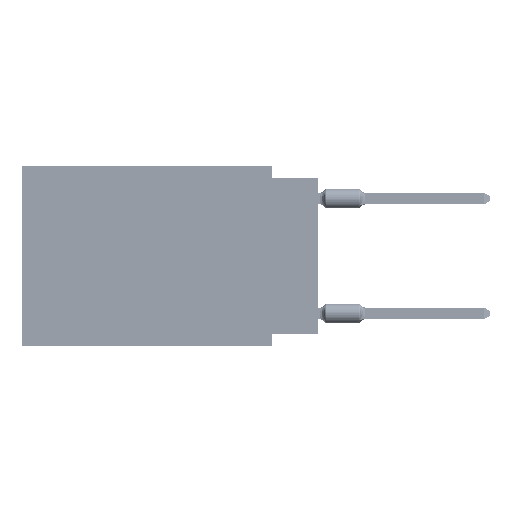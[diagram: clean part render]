
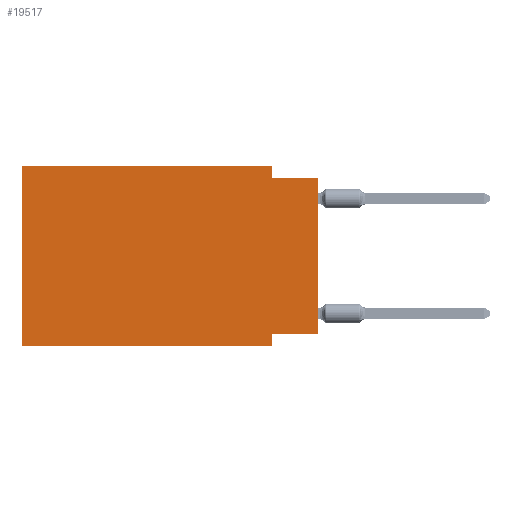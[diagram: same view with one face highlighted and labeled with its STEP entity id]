
A CAD part, left-side view. The second image highlights one B-rep face of the part: STEP entity #19517.
In plain terms, the highlighted planar face has unit normal (-1, 0, 0).
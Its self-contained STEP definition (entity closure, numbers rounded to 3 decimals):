
#997 = CARTESIAN_POINT ( 'NONE',  ( 0., 0., 0. ) ) ;
#1461 = ORIENTED_EDGE ( 'NONE', *, *, #12171, .T. ) ;
#1548 = CARTESIAN_POINT ( 'NONE',  ( 0., 16.383, 0. ) ) ;
#1754 = LINE ( 'NONE', #11423, #20943 ) ;
#3385 = VERTEX_POINT ( 'NONE', #8184 ) ;
#3868 = DIRECTION ( 'NONE',  ( 1., 0., 0. ) ) ;
#5602 = EDGE_CURVE ( 'NONE', #11889, #20168, #49366, .T. ) ;
#5923 = DIRECTION ( 'NONE',  ( 0., 1., 0. ) ) ;
#6121 = EDGE_CURVE ( 'NONE', #3385, #27417, #27793, .T. ) ;
#7916 = ORIENTED_EDGE ( 'NONE', *, *, #41001, .F. ) ;
#8184 = CARTESIAN_POINT ( 'NONE',  ( 0., 0., -9.271 ) ) ;
#9067 = CARTESIAN_POINT ( 'NONE',  ( 0., 16.383, 0. ) ) ;
#9395 = VECTOR ( 'NONE', #56361, 1000. ) ;
#11322 = VERTEX_POINT ( 'NONE', #67606 ) ;
#11423 = CARTESIAN_POINT ( 'NONE',  ( 0., 2.54, 0. ) ) ;
#11850 = CARTESIAN_POINT ( 'NONE',  ( 0., 0., -9.271 ) ) ;
#11889 = VERTEX_POINT ( 'NONE', #1548 ) ;
#12171 = EDGE_CURVE ( 'NONE', #3385, #71257, #22879, .T. ) ;
#13112 = VERTEX_POINT ( 'NONE', #24906 ) ;
#13745 = AXIS2_PLACEMENT_3D ( 'NONE', #41793, #3868, #64391 ) ;
#14829 = EDGE_CURVE ( 'NONE', #13112, #11889, #71295, .T. ) ;
#15281 = ORIENTED_EDGE ( 'NONE', *, *, #58398, .F. ) ;
#17285 = LINE ( 'NONE', #69511, #36307 ) ;
#18370 = DIRECTION ( 'NONE',  ( 0., 0., -1. ) ) ;
#19517 = ADVANCED_FACE ( 'NONE', ( #47333 ), #71661, .F. ) ;
#20168 = VERTEX_POINT ( 'NONE', #47807 ) ;
#20874 = CARTESIAN_POINT ( 'NONE',  ( 0., 16.383, 0. ) ) ;
#20943 = VECTOR ( 'NONE', #40680, 1000. ) ;
#22879 = LINE ( 'NONE', #997, #32936 ) ;
#23630 = CARTESIAN_POINT ( 'NONE',  ( 0., 0., -0.635 ) ) ;
#24906 = CARTESIAN_POINT ( 'NONE',  ( 0., 16.383, -9.906 ) ) ;
#26355 = VECTOR ( 'NONE', #65716, 1000. ) ;
#26816 = ORIENTED_EDGE ( 'NONE', *, *, #5602, .F. ) ;
#27417 = VERTEX_POINT ( 'NONE', #38513 ) ;
#27793 = LINE ( 'NONE', #11850, #51251 ) ;
#32936 = VECTOR ( 'NONE', #34378, 1000. ) ;
#34378 = DIRECTION ( 'NONE',  ( 0., 0., 1. ) ) ;
#36307 = VECTOR ( 'NONE', #68774, 1000. ) ;
#37496 = ORIENTED_EDGE ( 'NONE', *, *, #56570, .T. ) ;
#37605 = DIRECTION ( 'NONE',  ( 0., 0., 1. ) ) ;
#38513 = CARTESIAN_POINT ( 'NONE',  ( 0., 2.54, -9.271 ) ) ;
#40629 = LINE ( 'NONE', #69142, #43605 ) ;
#40680 = DIRECTION ( 'NONE',  ( 0., 0., -1. ) ) ;
#41001 = EDGE_CURVE ( 'NONE', #20168, #11322, #1754, .T. ) ;
#41793 = CARTESIAN_POINT ( 'NONE',  ( 0., 16.383, 0. ) ) ;
#43605 = VECTOR ( 'NONE', #18370, 1000. ) ;
#45502 = ORIENTED_EDGE ( 'NONE', *, *, #6121, .F. ) ;
#47333 = FACE_OUTER_BOUND ( 'NONE', #61001, .T. ) ;
#47807 = CARTESIAN_POINT ( 'NONE',  ( 0., 2.54, 0. ) ) ;
#49366 = LINE ( 'NONE', #20874, #26355 ) ;
#49898 = VECTOR ( 'NONE', #37605, 1000. ) ;
#50052 = CARTESIAN_POINT ( 'NONE',  ( 0., 16.383, -9.906 ) ) ;
#50950 = EDGE_CURVE ( 'NONE', #11322, #71257, #17285, .T. ) ;
#51251 = VECTOR ( 'NONE', #5923, 1000. ) ;
#52676 = ORIENTED_EDGE ( 'NONE', *, *, #50950, .F. ) ;
#56361 = DIRECTION ( 'NONE',  ( 0., -1., 0. ) ) ;
#56570 = EDGE_CURVE ( 'NONE', #13112, #58520, #73022, .T. ) ;
#58398 = EDGE_CURVE ( 'NONE', #27417, #58520, #40629, .T. ) ;
#58520 = VERTEX_POINT ( 'NONE', #69866 ) ;
#61001 = EDGE_LOOP ( 'NONE', ( #1461, #52676, #7916, #26816, #66743, #37496, #15281, #45502 ) ) ;
#64391 = DIRECTION ( 'NONE',  ( 0., 0., -1. ) ) ;
#65716 = DIRECTION ( 'NONE',  ( 0., -1., 0. ) ) ;
#66743 = ORIENTED_EDGE ( 'NONE', *, *, #14829, .F. ) ;
#67606 = CARTESIAN_POINT ( 'NONE',  ( 0., 2.54, -0.635 ) ) ;
#68774 = DIRECTION ( 'NONE',  ( 0., -1., 0. ) ) ;
#69142 = CARTESIAN_POINT ( 'NONE',  ( 0., 2.54, -9.906 ) ) ;
#69511 = CARTESIAN_POINT ( 'NONE',  ( 0., 0., -0.635 ) ) ;
#69866 = CARTESIAN_POINT ( 'NONE',  ( 0., 2.54, -9.906 ) ) ;
#71257 = VERTEX_POINT ( 'NONE', #23630 ) ;
#71295 = LINE ( 'NONE', #9067, #49898 ) ;
#71661 = PLANE ( 'NONE',  #13745 ) ;
#73022 = LINE ( 'NONE', #50052, #9395 ) ;
